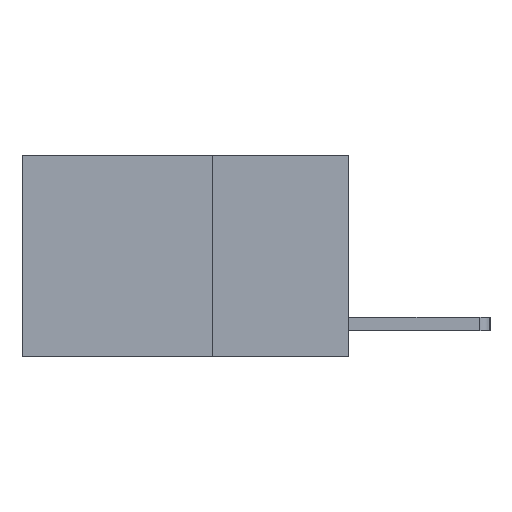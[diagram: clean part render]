
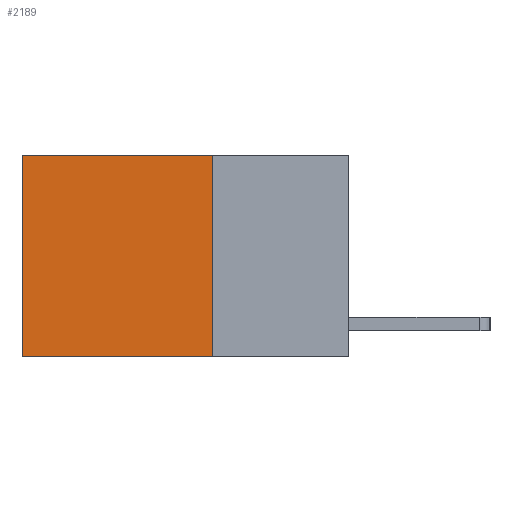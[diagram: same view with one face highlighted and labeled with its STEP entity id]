
A CAD part, left-side view. The second image highlights one B-rep face of the part: STEP entity #2189.
In plain terms, the highlighted planar face has unit normal (-1, 0, 0).
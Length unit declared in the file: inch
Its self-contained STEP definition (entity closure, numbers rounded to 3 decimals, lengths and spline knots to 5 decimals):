
#221 = VERTEX_POINT ( 'NONE', #862 ) ;
#314 = ORIENTED_EDGE ( 'NONE', *, *, #7391, .T. ) ;
#349 = VERTEX_POINT ( 'NONE', #466 ) ;
#466 = CARTESIAN_POINT ( 'NONE',  ( 0.2625, 0.6, 0. ) ) ;
#862 = CARTESIAN_POINT ( 'NONE',  ( 0.2625, 0.6, -0.37 ) ) ;
#1147 = VERTEX_POINT ( 'NONE', #7117 ) ;
#1765 = ORIENTED_EDGE ( 'NONE', *, *, #3460, .F. ) ;
#2094 = VECTOR ( 'NONE', #7122, 39.37008 ) ;
#2106 = LINE ( 'NONE', #6496, #2094 ) ;
#2189 = ADVANCED_FACE ( 'NONE', ( #5948 ), #4327, .F. ) ;
#2634 = AXIS2_PLACEMENT_3D ( 'NONE', #5171, #4123, #4040 ) ;
#3413 = EDGE_LOOP ( 'NONE', ( #314, #5869, #1765, #4263 ) ) ;
#3460 = EDGE_CURVE ( 'NONE', #8079, #1147, #7613, .T. ) ;
#3506 = DIRECTION ( 'NONE',  ( 0., 0., -1. ) ) ;
#3534 = VECTOR ( 'NONE', #8324, 39.37008 ) ;
#3633 = LINE ( 'NONE', #4515, #3534 ) ;
#3689 = EDGE_CURVE ( 'NONE', #1147, #221, #8128, .T. ) ;
#4040 = DIRECTION ( 'NONE',  ( 0., 0., -1. ) ) ;
#4123 = DIRECTION ( 'NONE',  ( 1., 0., 0. ) ) ;
#4263 = ORIENTED_EDGE ( 'NONE', *, *, #8406, .T. ) ;
#4327 = PLANE ( 'NONE',  #2634 ) ;
#4372 = CARTESIAN_POINT ( 'NONE',  ( 0.2625, 0.25, 0. ) ) ;
#4515 = CARTESIAN_POINT ( 'NONE',  ( 0.2625, 0.6, 0. ) ) ;
#4710 = VECTOR ( 'NONE', #3506, 39.37008 ) ;
#5024 = CARTESIAN_POINT ( 'NONE',  ( 0.2625, 0.25, 0. ) ) ;
#5171 = CARTESIAN_POINT ( 'NONE',  ( 0.2625, 0.25, 0. ) ) ;
#5869 = ORIENTED_EDGE ( 'NONE', *, *, #3689, .F. ) ;
#5948 = FACE_OUTER_BOUND ( 'NONE', #3413, .T. ) ;
#6496 = CARTESIAN_POINT ( 'NONE',  ( 0.2625, 0.25, 0. ) ) ;
#7117 = CARTESIAN_POINT ( 'NONE',  ( 0.2625, 0.25, -0.37 ) ) ;
#7122 = DIRECTION ( 'NONE',  ( 0., 1., 0. ) ) ;
#7391 = EDGE_CURVE ( 'NONE', #349, #221, #3633, .T. ) ;
#7515 = CARTESIAN_POINT ( 'NONE',  ( 0.2625, 0.25, -0.37 ) ) ;
#7521 = DIRECTION ( 'NONE',  ( 0., 1., 0. ) ) ;
#7613 = LINE ( 'NONE', #5024, #4710 ) ;
#8079 = VERTEX_POINT ( 'NONE', #4372 ) ;
#8128 = LINE ( 'NONE', #7515, #8199 ) ;
#8199 = VECTOR ( 'NONE', #7521, 39.37008 ) ;
#8324 = DIRECTION ( 'NONE',  ( 0., 0., -1. ) ) ;
#8406 = EDGE_CURVE ( 'NONE', #8079, #349, #2106, .T. ) ;
